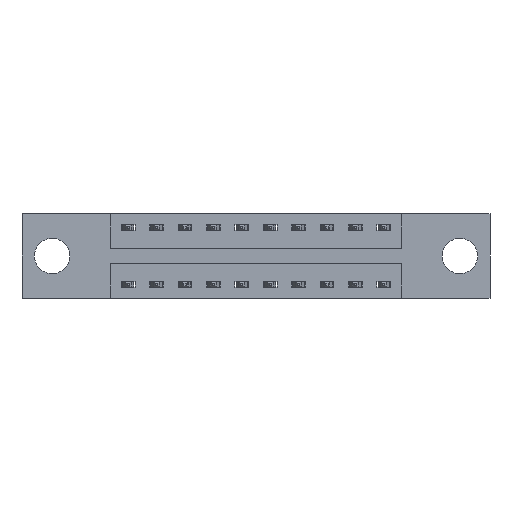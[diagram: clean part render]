
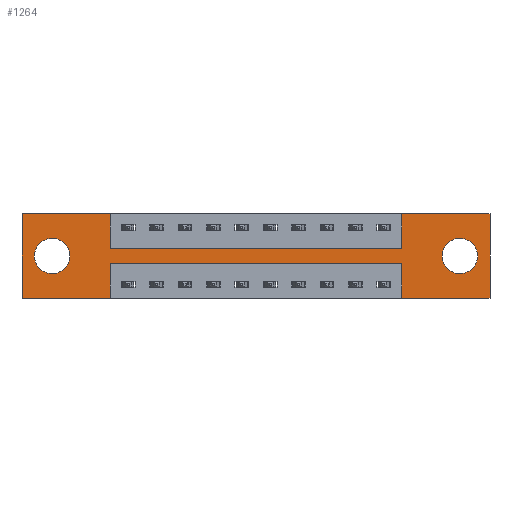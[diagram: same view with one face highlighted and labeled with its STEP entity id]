
A CAD part, front view. The second image highlights one B-rep face of the part: STEP entity #1264.
In plain terms, the highlighted planar face has unit normal (0, -1, 0).
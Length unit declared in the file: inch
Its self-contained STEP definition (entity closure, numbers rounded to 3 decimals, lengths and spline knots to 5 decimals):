
#101 = CARTESIAN_POINT ( 'NONE',  ( 0.3875, 0., -0.22 ) ) ;
#105 = FACE_OUTER_BOUND ( 'NONE', #1944, .T. ) ;
#113 = ORIENTED_EDGE ( 'NONE', *, *, #3605, .F. ) ;
#278 = VERTEX_POINT ( 'NONE', #1344 ) ;
#544 = EDGE_CURVE ( 'NONE', #1584, #9357, #9063, .T. ) ;
#565 = EDGE_CURVE ( 'NONE', #1591, #7112, #6049, .T. ) ;
#573 = CARTESIAN_POINT ( 'NONE',  ( 0., 0., 0. ) ) ;
#677 = EDGE_CURVE ( 'NONE', #2299, #5138, #3952, .T. ) ;
#735 = CARTESIAN_POINT ( 'NONE',  ( 0., 0., -0.37 ) ) ;
#742 = CARTESIAN_POINT ( 'NONE',  ( 1.9275, 0., -0.185 ) ) ;
#750 = VERTEX_POINT ( 'NONE', #6708 ) ;
#842 = CARTESIAN_POINT ( 'NONE',  ( 0., 0., 0. ) ) ;
#999 = CARTESIAN_POINT ( 'NONE',  ( 0.3875, 0., -0.37 ) ) ;
#1226 = ORIENTED_EDGE ( 'NONE', *, *, #2967, .F. ) ;
#1242 = DIRECTION ( 'NONE',  ( 0., 0., 1. ) ) ;
#1243 = DIRECTION ( 'NONE',  ( -1., 0., 0. ) ) ;
#1264 = ADVANCED_FACE ( 'NONE', ( #8909, #1537, #105 ), #4842, .T. ) ;
#1344 = CARTESIAN_POINT ( 'NONE',  ( 0.1325, 0., -0.107 ) ) ;
#1410 = CARTESIAN_POINT ( 'NONE',  ( 0., 0., -0.37 ) ) ;
#1437 = ORIENTED_EDGE ( 'NONE', *, *, #10651, .F. ) ;
#1446 = CARTESIAN_POINT ( 'NONE',  ( 0.3875, 0., -0.15 ) ) ;
#1495 = DIRECTION ( 'NONE',  ( 0., 0., 1. ) ) ;
#1515 = DIRECTION ( 'NONE',  ( 0., 0., 1. ) ) ;
#1537 = FACE_BOUND ( 'NONE', #7277, .T. ) ;
#1584 = VERTEX_POINT ( 'NONE', #2422 ) ;
#1591 = VERTEX_POINT ( 'NONE', #10849 ) ;
#1596 = EDGE_CURVE ( 'NONE', #750, #1591, #9942, .T. ) ;
#1671 = DIRECTION ( 'NONE',  ( 0., 1., 0. ) ) ;
#1944 = EDGE_LOOP ( 'NONE', ( #4163, #6662, #2986, #8814, #9654, #7034, #1226, #1437, #6421, #2858, #113, #5749 ) ) ;
#2215 = VECTOR ( 'NONE', #4162, 39.37008 ) ;
#2299 = VERTEX_POINT ( 'NONE', #999 ) ;
#2346 = CARTESIAN_POINT ( 'NONE',  ( 1.6725, 0., -0.22 ) ) ;
#2422 = CARTESIAN_POINT ( 'NONE',  ( 1.9275, 0., -0.107 ) ) ;
#2462 = EDGE_CURVE ( 'NONE', #4647, #3520, #6259, .T. ) ;
#2542 = CIRCLE ( 'NONE', #4606, 0.078 ) ;
#2666 = CIRCLE ( 'NONE', #6292, 0.078 ) ;
#2786 = CARTESIAN_POINT ( 'NONE',  ( 0.1325, 0., -0.185 ) ) ;
#2811 = LINE ( 'NONE', #9125, #4133 ) ;
#2854 = DIRECTION ( 'NONE',  ( 0., 1., 0. ) ) ;
#2858 = ORIENTED_EDGE ( 'NONE', *, *, #9185, .F. ) ;
#2902 = CARTESIAN_POINT ( 'NONE',  ( 1.6725, 0., 0. ) ) ;
#2906 = ORIENTED_EDGE ( 'NONE', *, *, #10733, .T. ) ;
#2967 = EDGE_CURVE ( 'NONE', #4012, #750, #8734, .T. ) ;
#2986 = ORIENTED_EDGE ( 'NONE', *, *, #6140, .F. ) ;
#3057 = AXIS2_PLACEMENT_3D ( 'NONE', #742, #1671, #8395 ) ;
#3075 = CARTESIAN_POINT ( 'NONE',  ( 0., 0., -0.37 ) ) ;
#3091 = VECTOR ( 'NONE', #1242, 39.37008 ) ;
#3511 = CARTESIAN_POINT ( 'NONE',  ( 1.9275, 0., -0.185 ) ) ;
#3520 = VERTEX_POINT ( 'NONE', #5953 ) ;
#3571 = CIRCLE ( 'NONE', #5770, 0.078 ) ;
#3580 = DIRECTION ( 'NONE',  ( 0., 0., 1. ) ) ;
#3586 = CARTESIAN_POINT ( 'NONE',  ( 0.3875, 0., 0. ) ) ;
#3605 = EDGE_CURVE ( 'NONE', #5138, #5428, #2811, .T. ) ;
#3764 = CARTESIAN_POINT ( 'NONE',  ( 0.1325, 0., -0.263 ) ) ;
#3952 = LINE ( 'NONE', #1410, #10240 ) ;
#4012 = VERTEX_POINT ( 'NONE', #7819 ) ;
#4038 = VECTOR ( 'NONE', #1243, 39.37008 ) ;
#4043 = DIRECTION ( 'NONE',  ( 0., -1., 0. ) ) ;
#4045 = CARTESIAN_POINT ( 'NONE',  ( 0.3875, 0., 0. ) ) ;
#4133 = VECTOR ( 'NONE', #1495, 39.37008 ) ;
#4162 = DIRECTION ( 'NONE',  ( 0., 0., -1. ) ) ;
#4163 = ORIENTED_EDGE ( 'NONE', *, *, #8542, .F. ) ;
#4320 = DIRECTION ( 'NONE',  ( 0., 0., -1. ) ) ;
#4606 = AXIS2_PLACEMENT_3D ( 'NONE', #8114, #7713, #7642 ) ;
#4647 = VERTEX_POINT ( 'NONE', #2346 ) ;
#4802 = DIRECTION ( 'NONE',  ( 1., 0., 0. ) ) ;
#4842 = PLANE ( 'NONE',  #9516 ) ;
#4895 = EDGE_CURVE ( 'NONE', #8209, #278, #3571, .T. ) ;
#5017 = DIRECTION ( 'NONE',  ( 1., 0., 0. ) ) ;
#5071 = DIRECTION ( 'NONE',  ( 0., 0., -1. ) ) ;
#5084 = DIRECTION ( 'NONE',  ( -1., 0., 0. ) ) ;
#5138 = VERTEX_POINT ( 'NONE', #735 ) ;
#5192 = DIRECTION ( 'NONE',  ( 0., 1., 0. ) ) ;
#5300 = VERTEX_POINT ( 'NONE', #10120 ) ;
#5428 = VERTEX_POINT ( 'NONE', #573 ) ;
#5596 = VERTEX_POINT ( 'NONE', #7551 ) ;
#5660 = EDGE_CURVE ( 'NONE', #9357, #1584, #2666, .T. ) ;
#5749 = ORIENTED_EDGE ( 'NONE', *, *, #677, .F. ) ;
#5770 = AXIS2_PLACEMENT_3D ( 'NONE', #2786, #2854, #3580 ) ;
#5889 = CARTESIAN_POINT ( 'NONE',  ( 0., 0., 0. ) ) ;
#5953 = CARTESIAN_POINT ( 'NONE',  ( 0.3875, 0., -0.22 ) ) ;
#6049 = LINE ( 'NONE', #7452, #2215 ) ;
#6100 = LINE ( 'NONE', #1446, #6621 ) ;
#6140 = EDGE_CURVE ( 'NONE', #5300, #4647, #6833, .T. ) ;
#6259 = LINE ( 'NONE', #101, #10436 ) ;
#6261 = LINE ( 'NONE', #9601, #4038 ) ;
#6292 = AXIS2_PLACEMENT_3D ( 'NONE', #3511, #5192, #10051 ) ;
#6397 = LINE ( 'NONE', #6929, #10443 ) ;
#6421 = ORIENTED_EDGE ( 'NONE', *, *, #9297, .F. ) ;
#6516 = VECTOR ( 'NONE', #9425, 39.37008 ) ;
#6621 = VECTOR ( 'NONE', #4802, 39.37008 ) ;
#6662 = ORIENTED_EDGE ( 'NONE', *, *, #2462, .F. ) ;
#6708 = CARTESIAN_POINT ( 'NONE',  ( 1.6725, 0., 0. ) ) ;
#6711 = VERTEX_POINT ( 'NONE', #4045 ) ;
#6833 = LINE ( 'NONE', #8313, #10608 ) ;
#6929 = CARTESIAN_POINT ( 'NONE',  ( 0.3875, 0., -0.37 ) ) ;
#7004 = CARTESIAN_POINT ( 'NONE',  ( 2.06, 0., -0.37 ) ) ;
#7034 = ORIENTED_EDGE ( 'NONE', *, *, #1596, .F. ) ;
#7112 = VERTEX_POINT ( 'NONE', #7004 ) ;
#7208 = VECTOR ( 'NONE', #5017, 39.37008 ) ;
#7277 = EDGE_LOOP ( 'NONE', ( #2906, #9334 ) ) ;
#7357 = DIRECTION ( 'NONE',  ( -1., 0., 0. ) ) ;
#7429 = LINE ( 'NONE', #842, #6516 ) ;
#7452 = CARTESIAN_POINT ( 'NONE',  ( 2.06, 0., 0. ) ) ;
#7551 = CARTESIAN_POINT ( 'NONE',  ( 0.3875, 0., -0.15 ) ) ;
#7642 = DIRECTION ( 'NONE',  ( 0., 0., 1. ) ) ;
#7698 = LINE ( 'NONE', #3586, #8870 ) ;
#7713 = DIRECTION ( 'NONE',  ( 0., 1., 0. ) ) ;
#7733 = DIRECTION ( 'NONE',  ( 0., 0., -1. ) ) ;
#7819 = CARTESIAN_POINT ( 'NONE',  ( 1.6725, 0., -0.15 ) ) ;
#8114 = CARTESIAN_POINT ( 'NONE',  ( 0.1325, 0., -0.185 ) ) ;
#8209 = VERTEX_POINT ( 'NONE', #3764 ) ;
#8313 = CARTESIAN_POINT ( 'NONE',  ( 1.6725, 0., -0.37 ) ) ;
#8395 = DIRECTION ( 'NONE',  ( 0., 0., -1. ) ) ;
#8465 = ORIENTED_EDGE ( 'NONE', *, *, #544, .T. ) ;
#8542 = EDGE_CURVE ( 'NONE', #3520, #2299, #6397, .T. ) ;
#8676 = CARTESIAN_POINT ( 'NONE',  ( 1.9275, 0., -0.263 ) ) ;
#8734 = LINE ( 'NONE', #2902, #3091 ) ;
#8814 = ORIENTED_EDGE ( 'NONE', *, *, #9319, .F. ) ;
#8870 = VECTOR ( 'NONE', #4320, 39.37008 ) ;
#8909 = FACE_BOUND ( 'NONE', #9450, .T. ) ;
#9063 = CIRCLE ( 'NONE', #3057, 0.078 ) ;
#9076 = ORIENTED_EDGE ( 'NONE', *, *, #5660, .T. ) ;
#9125 = CARTESIAN_POINT ( 'NONE',  ( 0., 0., 0. ) ) ;
#9185 = EDGE_CURVE ( 'NONE', #5428, #6711, #7429, .T. ) ;
#9297 = EDGE_CURVE ( 'NONE', #6711, #5596, #7698, .T. ) ;
#9319 = EDGE_CURVE ( 'NONE', #7112, #5300, #6261, .T. ) ;
#9334 = ORIENTED_EDGE ( 'NONE', *, *, #4895, .T. ) ;
#9357 = VERTEX_POINT ( 'NONE', #8676 ) ;
#9425 = DIRECTION ( 'NONE',  ( 1., 0., 0. ) ) ;
#9450 = EDGE_LOOP ( 'NONE', ( #8465, #9076 ) ) ;
#9516 = AXIS2_PLACEMENT_3D ( 'NONE', #3075, #4043, #5071 ) ;
#9601 = CARTESIAN_POINT ( 'NONE',  ( 0., 0., -0.37 ) ) ;
#9654 = ORIENTED_EDGE ( 'NONE', *, *, #565, .F. ) ;
#9942 = LINE ( 'NONE', #5889, #7208 ) ;
#10051 = DIRECTION ( 'NONE',  ( 0., 0., -1. ) ) ;
#10120 = CARTESIAN_POINT ( 'NONE',  ( 1.6725, 0., -0.37 ) ) ;
#10240 = VECTOR ( 'NONE', #7357, 39.37008 ) ;
#10436 = VECTOR ( 'NONE', #5084, 39.37008 ) ;
#10443 = VECTOR ( 'NONE', #7733, 39.37008 ) ;
#10608 = VECTOR ( 'NONE', #1515, 39.37008 ) ;
#10651 = EDGE_CURVE ( 'NONE', #5596, #4012, #6100, .T. ) ;
#10733 = EDGE_CURVE ( 'NONE', #278, #8209, #2542, .T. ) ;
#10849 = CARTESIAN_POINT ( 'NONE',  ( 2.06, 0., 0. ) ) ;
